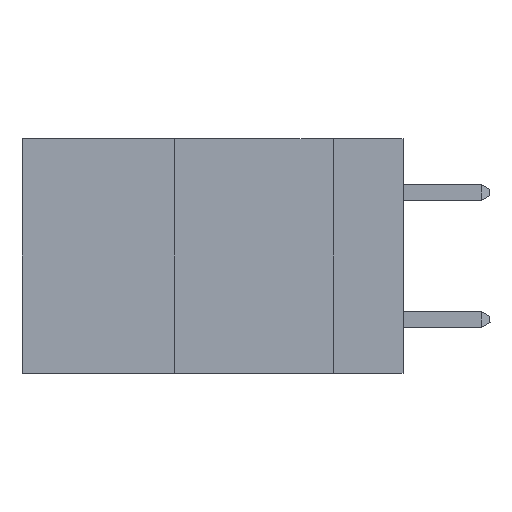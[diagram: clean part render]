
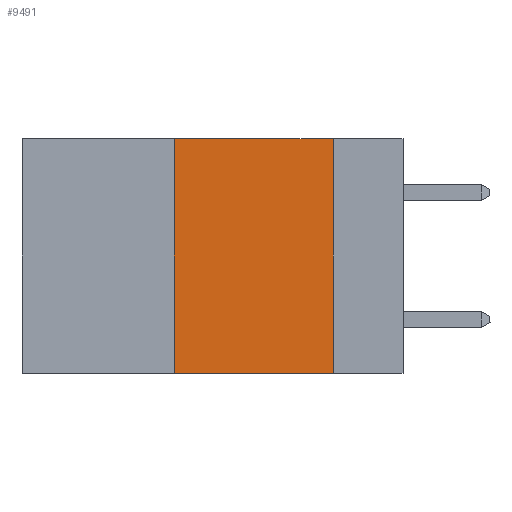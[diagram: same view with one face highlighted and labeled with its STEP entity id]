
A CAD part, left-side view. The second image highlights one B-rep face of the part: STEP entity #9491.
In plain terms, the highlighted planar face has unit normal (-1, 0, 0).
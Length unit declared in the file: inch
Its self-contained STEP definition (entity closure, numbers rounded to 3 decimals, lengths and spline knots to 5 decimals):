
#1607 = EDGE_CURVE ( 'NONE', #17660, #26779, #8064, .T. ) ;
#2110 = EDGE_CURVE ( 'NONE', #8282, #23215, #18831, .T. ) ;
#3520 = DIRECTION ( 'NONE',  ( 0., 0., 1. ) ) ;
#3742 = CARTESIAN_POINT ( 'NONE',  ( 0., 0.6, 0. ) ) ;
#3971 = CARTESIAN_POINT ( 'NONE',  ( 0., 0.36, 0. ) ) ;
#5987 = CARTESIAN_POINT ( 'NONE',  ( 0., 0.11, 0. ) ) ;
#7336 = VECTOR ( 'NONE', #10912, 39.37008 ) ;
#8064 = LINE ( 'NONE', #8607, #7336 ) ;
#8282 = VERTEX_POINT ( 'NONE', #3971 ) ;
#8356 = DIRECTION ( 'NONE',  ( 0., 0., -1. ) ) ;
#8607 = CARTESIAN_POINT ( 'NONE',  ( 0., 0.6, -0.37 ) ) ;
#9491 = ADVANCED_FACE ( 'NONE', ( #10761 ), #19832, .F. ) ;
#10761 = FACE_OUTER_BOUND ( 'NONE', #26057, .T. ) ;
#10912 = DIRECTION ( 'NONE',  ( 0., -1., 0. ) ) ;
#11613 = VECTOR ( 'NONE', #3520, 39.37008 ) ;
#12804 = DIRECTION ( 'NONE',  ( 0., 0., -1. ) ) ;
#15114 = EDGE_CURVE ( 'NONE', #23215, #26779, #15243, .T. ) ;
#15243 = LINE ( 'NONE', #5987, #20643 ) ;
#15350 = ORIENTED_EDGE ( 'NONE', *, *, #2110, .F. ) ;
#15612 = CARTESIAN_POINT ( 'NONE',  ( 0., 0.36, -0.37 ) ) ;
#15715 = ORIENTED_EDGE ( 'NONE', *, *, #29175, .F. ) ;
#17660 = VERTEX_POINT ( 'NONE', #15612 ) ;
#18108 = VECTOR ( 'NONE', #21654, 39.37008 ) ;
#18715 = AXIS2_PLACEMENT_3D ( 'NONE', #3742, #22136, #8356 ) ;
#18831 = LINE ( 'NONE', #19335, #18108 ) ;
#19335 = CARTESIAN_POINT ( 'NONE',  ( 0., 0.6, 0. ) ) ;
#19832 = PLANE ( 'NONE',  #18715 ) ;
#20643 = VECTOR ( 'NONE', #12804, 39.37008 ) ;
#21654 = DIRECTION ( 'NONE',  ( 0., -1., 0. ) ) ;
#21926 = CARTESIAN_POINT ( 'NONE',  ( 0., 0.36, 0. ) ) ;
#22136 = DIRECTION ( 'NONE',  ( 1., 0., 0. ) ) ;
#22674 = CARTESIAN_POINT ( 'NONE',  ( 0., 0.11, 0. ) ) ;
#23215 = VERTEX_POINT ( 'NONE', #22674 ) ;
#23869 = LINE ( 'NONE', #21926, #11613 ) ;
#25755 = ORIENTED_EDGE ( 'NONE', *, *, #1607, .T. ) ;
#26057 = EDGE_LOOP ( 'NONE', ( #29499, #15350, #15715, #25755 ) ) ;
#26779 = VERTEX_POINT ( 'NONE', #27049 ) ;
#27049 = CARTESIAN_POINT ( 'NONE',  ( 0., 0.11, -0.37 ) ) ;
#29175 = EDGE_CURVE ( 'NONE', #17660, #8282, #23869, .T. ) ;
#29499 = ORIENTED_EDGE ( 'NONE', *, *, #15114, .F. ) ;
